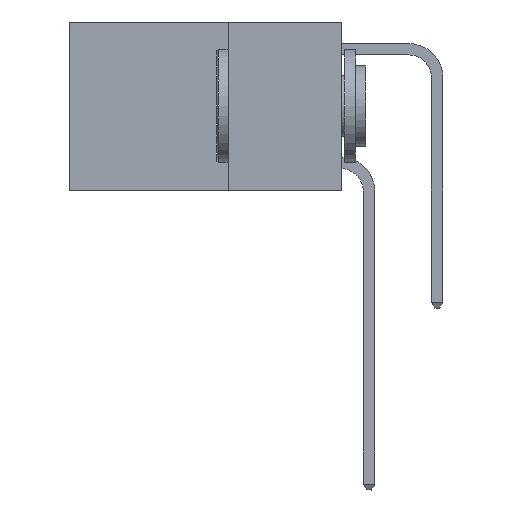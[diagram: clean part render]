
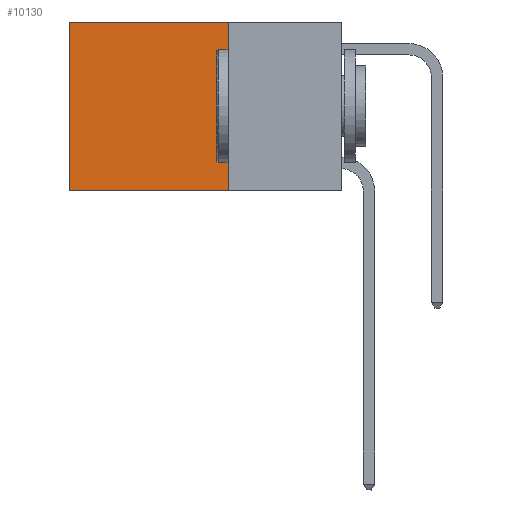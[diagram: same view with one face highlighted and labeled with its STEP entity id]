
A CAD part, left-side view. The second image highlights one B-rep face of the part: STEP entity #10130.
In plain terms, the highlighted planar face has unit normal (-1, 0, 0).
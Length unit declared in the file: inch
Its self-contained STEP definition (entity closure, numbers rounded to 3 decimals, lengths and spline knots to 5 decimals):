
#722 = CARTESIAN_POINT ( 'NONE',  ( 0.2625, 0.6, 0. ) ) ;
#1107 = DIRECTION ( 'NONE',  ( 1., 0., 0. ) ) ;
#1114 = LINE ( 'NONE', #12685, #4867 ) ;
#1534 = AXIS2_PLACEMENT_3D ( 'NONE', #12959, #1107, #6964 ) ;
#2045 = CARTESIAN_POINT ( 'NONE',  ( 0.2625, 0.25, -0.37 ) ) ;
#2160 = EDGE_CURVE ( 'NONE', #19206, #9880, #12905, .T. ) ;
#2161 = EDGE_CURVE ( 'NONE', #13280, #2764, #7700, .T. ) ;
#2764 = VERTEX_POINT ( 'NONE', #722 ) ;
#3052 = CARTESIAN_POINT ( 'NONE',  ( 0.2625, 0.25, 0. ) ) ;
#3530 = FACE_OUTER_BOUND ( 'NONE', #14245, .T. ) ;
#3878 = LINE ( 'NONE', #17032, #19432 ) ;
#4414 = EDGE_CURVE ( 'NONE', #13280, #19206, #3878, .T. ) ;
#4867 = VECTOR ( 'NONE', #17264, 39.37008 ) ;
#6341 = ORIENTED_EDGE ( 'NONE', *, *, #4414, .F. ) ;
#6657 = ORIENTED_EDGE ( 'NONE', *, *, #2161, .T. ) ;
#6964 = DIRECTION ( 'NONE',  ( 0., 0., -1. ) ) ;
#7616 = ORIENTED_EDGE ( 'NONE', *, *, #11827, .T. ) ;
#7700 = LINE ( 'NONE', #15747, #14318 ) ;
#8864 = VECTOR ( 'NONE', #15675, 39.37008 ) ;
#9880 = VERTEX_POINT ( 'NONE', #11379 ) ;
#10090 = ORIENTED_EDGE ( 'NONE', *, *, #2160, .F. ) ;
#10130 = ADVANCED_FACE ( 'NONE', ( #3530 ), #14591, .F. ) ;
#10169 = DIRECTION ( 'NONE',  ( 0., 1., 0. ) ) ;
#11379 = CARTESIAN_POINT ( 'NONE',  ( 0.2625, 0.6, -0.37 ) ) ;
#11827 = EDGE_CURVE ( 'NONE', #2764, #9880, #1114, .T. ) ;
#12685 = CARTESIAN_POINT ( 'NONE',  ( 0.2625, 0.6, 0. ) ) ;
#12905 = LINE ( 'NONE', #2045, #8864 ) ;
#12959 = CARTESIAN_POINT ( 'NONE',  ( 0.2625, 0.25, 0. ) ) ;
#13280 = VERTEX_POINT ( 'NONE', #3052 ) ;
#14245 = EDGE_LOOP ( 'NONE', ( #7616, #10090, #6341, #6657 ) ) ;
#14318 = VECTOR ( 'NONE', #10169, 39.37008 ) ;
#14591 = PLANE ( 'NONE',  #1534 ) ;
#14996 = CARTESIAN_POINT ( 'NONE',  ( 0.2625, 0.25, -0.37 ) ) ;
#15489 = DIRECTION ( 'NONE',  ( 0., 0., -1. ) ) ;
#15675 = DIRECTION ( 'NONE',  ( 0., 1., 0. ) ) ;
#15747 = CARTESIAN_POINT ( 'NONE',  ( 0.2625, 0.25, 0. ) ) ;
#17032 = CARTESIAN_POINT ( 'NONE',  ( 0.2625, 0.25, 0. ) ) ;
#17264 = DIRECTION ( 'NONE',  ( 0., 0., -1. ) ) ;
#19206 = VERTEX_POINT ( 'NONE', #14996 ) ;
#19432 = VECTOR ( 'NONE', #15489, 39.37008 ) ;
